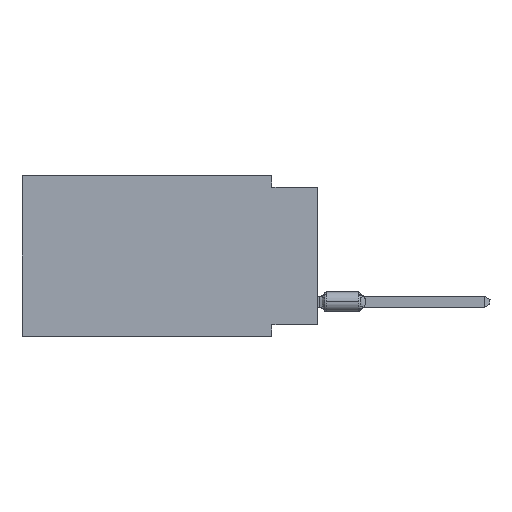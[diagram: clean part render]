
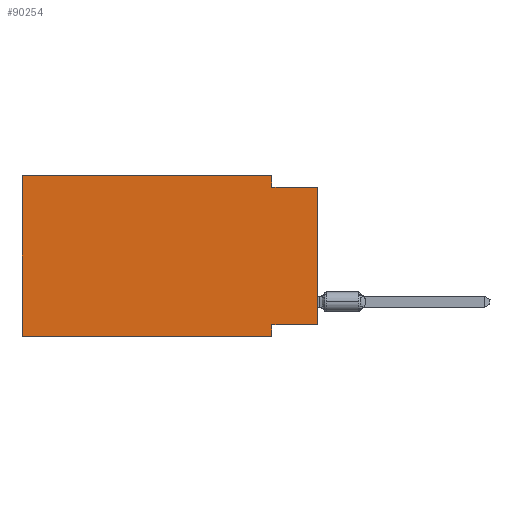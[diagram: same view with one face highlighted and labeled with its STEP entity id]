
A CAD part, left-side view. The second image highlights one B-rep face of the part: STEP entity #90254.
In plain terms, the highlighted planar face has unit normal (-1, 0, 0).
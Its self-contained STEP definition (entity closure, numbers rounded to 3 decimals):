
#9190 = ORIENTED_EDGE ( 'NONE', *, *, #32191, .F. ) ;
#9920 = CARTESIAN_POINT ( 'NONE',  ( 0., 0., 0. ) ) ;
#9987 = FACE_OUTER_BOUND ( 'NONE', #32706, .T. ) ;
#10239 = ORIENTED_EDGE ( 'NONE', *, *, #18047, .F. ) ;
#11801 = VECTOR ( 'NONE', #58291, 1000. ) ;
#13125 = DIRECTION ( 'NONE',  ( 0., 1., 0. ) ) ;
#13441 = EDGE_CURVE ( 'NONE', #42611, #36734, #52819, .T. ) ;
#14573 = ORIENTED_EDGE ( 'NONE', *, *, #13441, .T. ) ;
#15237 = DIRECTION ( 'NONE',  ( 0., 0., -1. ) ) ;
#18047 = EDGE_CURVE ( 'NONE', #73121, #33682, #87138, .T. ) ;
#20350 = VECTOR ( 'NONE', #51453, 1000. ) ;
#22814 = ORIENTED_EDGE ( 'NONE', *, *, #97671, .F. ) ;
#23115 = LINE ( 'NONE', #40158, #11801 ) ;
#24885 = PLANE ( 'NONE',  #29905 ) ;
#29905 = AXIS2_PLACEMENT_3D ( 'NONE', #83711, #58435, #49644 ) ;
#30582 = LINE ( 'NONE', #98185, #100756 ) ;
#30744 = VECTOR ( 'NONE', #15237, 1000. ) ;
#32191 = EDGE_CURVE ( 'NONE', #42611, #42338, #71423, .T. ) ;
#32706 = EDGE_LOOP ( 'NONE', ( #14573, #22814, #80684, #10239, #67870, #81928, #87052, #9190 ) ) ;
#33682 = VERTEX_POINT ( 'NONE', #57791 ) ;
#35351 = EDGE_CURVE ( 'NONE', #42338, #52727, #97737, .T. ) ;
#35760 = DIRECTION ( 'NONE',  ( 0., 0., 1. ) ) ;
#36324 = VECTOR ( 'NONE', #70440, 1000. ) ;
#36572 = CARTESIAN_POINT ( 'NONE',  ( 0., 16.383, 0. ) ) ;
#36734 = VERTEX_POINT ( 'NONE', #92362 ) ;
#37065 = CARTESIAN_POINT ( 'NONE',  ( 0., 2.54, 0. ) ) ;
#37434 = CARTESIAN_POINT ( 'NONE',  ( 0., 16.383, -8.89 ) ) ;
#40158 = CARTESIAN_POINT ( 'NONE',  ( 0., 16.383, 0. ) ) ;
#42338 = VERTEX_POINT ( 'NONE', #78774 ) ;
#42611 = VERTEX_POINT ( 'NONE', #51198 ) ;
#43086 = EDGE_CURVE ( 'NONE', #33682, #98113, #77389, .T. ) ;
#46149 = CARTESIAN_POINT ( 'NONE',  ( 0., 0., -8.255 ) ) ;
#49644 = DIRECTION ( 'NONE',  ( 0., 0., -1. ) ) ;
#51198 = CARTESIAN_POINT ( 'NONE',  ( 0., 0., -8.255 ) ) ;
#51453 = DIRECTION ( 'NONE',  ( 0., -1., 0. ) ) ;
#52727 = VERTEX_POINT ( 'NONE', #73314 ) ;
#52819 = LINE ( 'NONE', #9920, #72510 ) ;
#53394 = DIRECTION ( 'NONE',  ( 0., 0., -1. ) ) ;
#57791 = CARTESIAN_POINT ( 'NONE',  ( 0., 2.54, 0. ) ) ;
#58291 = DIRECTION ( 'NONE',  ( 0., 0., 1. ) ) ;
#58435 = DIRECTION ( 'NONE',  ( 1., 0., 0. ) ) ;
#62562 = VERTEX_POINT ( 'NONE', #65199 ) ;
#65199 = CARTESIAN_POINT ( 'NONE',  ( 0., 16.383, -8.89 ) ) ;
#66184 = EDGE_CURVE ( 'NONE', #62562, #52727, #103410, .T. ) ;
#67870 = ORIENTED_EDGE ( 'NONE', *, *, #103315, .F. ) ;
#70440 = DIRECTION ( 'NONE',  ( 0., -1., 0. ) ) ;
#71423 = LINE ( 'NONE', #46149, #95166 ) ;
#72510 = VECTOR ( 'NONE', #35760, 1000. ) ;
#73121 = VERTEX_POINT ( 'NONE', #96663 ) ;
#73314 = CARTESIAN_POINT ( 'NONE',  ( 0., 2.54, -8.89 ) ) ;
#77389 = LINE ( 'NONE', #37065, #93324 ) ;
#78774 = CARTESIAN_POINT ( 'NONE',  ( 0., 2.54, -8.255 ) ) ;
#80684 = ORIENTED_EDGE ( 'NONE', *, *, #43086, .F. ) ;
#81269 = CARTESIAN_POINT ( 'NONE',  ( 0., 2.54, -8.89 ) ) ;
#81928 = ORIENTED_EDGE ( 'NONE', *, *, #66184, .T. ) ;
#83711 = CARTESIAN_POINT ( 'NONE',  ( 0., 16.383, 0. ) ) ;
#87052 = ORIENTED_EDGE ( 'NONE', *, *, #35351, .F. ) ;
#87138 = LINE ( 'NONE', #36572, #20350 ) ;
#90254 = ADVANCED_FACE ( 'NONE', ( #9987 ), #24885, .F. ) ;
#91035 = DIRECTION ( 'NONE',  ( 0., -1., 0. ) ) ;
#92362 = CARTESIAN_POINT ( 'NONE',  ( 0., 0., -0.635 ) ) ;
#93324 = VECTOR ( 'NONE', #53394, 1000. ) ;
#95166 = VECTOR ( 'NONE', #13125, 1000. ) ;
#96293 = CARTESIAN_POINT ( 'NONE',  ( 0., 2.54, -0.635 ) ) ;
#96663 = CARTESIAN_POINT ( 'NONE',  ( 0., 16.383, 0. ) ) ;
#97671 = EDGE_CURVE ( 'NONE', #98113, #36734, #30582, .T. ) ;
#97737 = LINE ( 'NONE', #81269, #30744 ) ;
#98113 = VERTEX_POINT ( 'NONE', #96293 ) ;
#98185 = CARTESIAN_POINT ( 'NONE',  ( 0., 0., -0.635 ) ) ;
#100756 = VECTOR ( 'NONE', #91035, 1000. ) ;
#103315 = EDGE_CURVE ( 'NONE', #62562, #73121, #23115, .T. ) ;
#103410 = LINE ( 'NONE', #37434, #36324 ) ;
